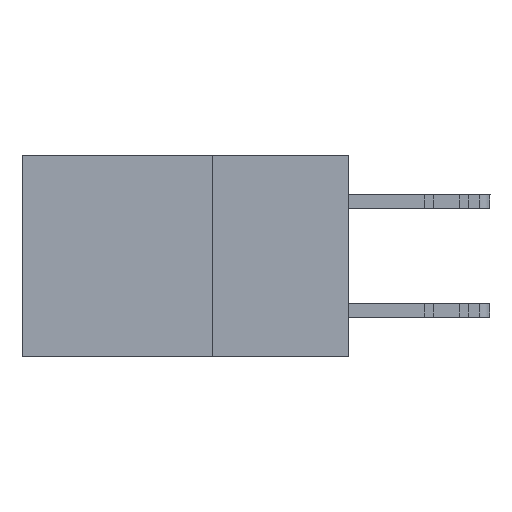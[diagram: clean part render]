
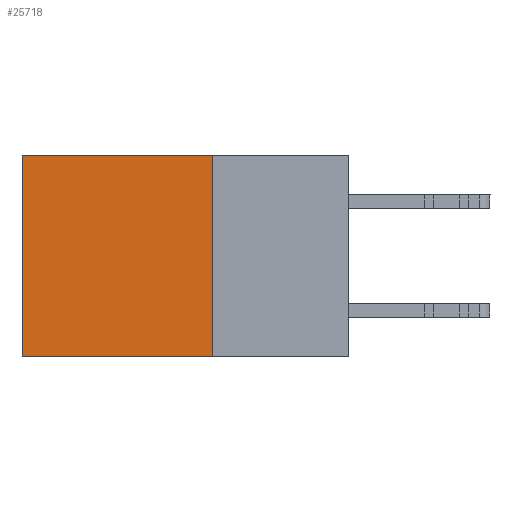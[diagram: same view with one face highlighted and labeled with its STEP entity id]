
A CAD part, left-side view. The second image highlights one B-rep face of the part: STEP entity #25718.
In plain terms, the highlighted planar face has unit normal (-1, 0, 0).
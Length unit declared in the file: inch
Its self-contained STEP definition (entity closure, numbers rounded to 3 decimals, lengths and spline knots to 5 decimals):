
#1016 = DIRECTION ( 'NONE',  ( 0., 0., -1. ) ) ;
#1740 = LINE ( 'NONE', #15560, #11359 ) ;
#2444 = EDGE_CURVE ( 'NONE', #27119, #6983, #7202, .T. ) ;
#3487 = DIRECTION ( 'NONE',  ( 0., 0., -1. ) ) ;
#3711 = ORIENTED_EDGE ( 'NONE', *, *, #20367, .T. ) ;
#4705 = EDGE_CURVE ( 'NONE', #25861, #27119, #5839, .T. ) ;
#5003 = FACE_OUTER_BOUND ( 'NONE', #18993, .T. ) ;
#5608 = VECTOR ( 'NONE', #3487, 39.37008 ) ;
#5630 = CARTESIAN_POINT ( 'NONE',  ( 0.298, 0.6, -0.37 ) ) ;
#5839 = LINE ( 'NONE', #16760, #5608 ) ;
#6544 = CARTESIAN_POINT ( 'NONE',  ( 0.298, 0.6, 0. ) ) ;
#6946 = CARTESIAN_POINT ( 'NONE',  ( 0.298, 0.25, 0. ) ) ;
#6983 = VERTEX_POINT ( 'NONE', #5630 ) ;
#7202 = LINE ( 'NONE', #20782, #8450 ) ;
#7620 = LINE ( 'NONE', #20776, #29014 ) ;
#8450 = VECTOR ( 'NONE', #11633, 39.37008 ) ;
#9418 = ORIENTED_EDGE ( 'NONE', *, *, #4705, .F. ) ;
#9603 = DIRECTION ( 'NONE',  ( 1., 0., 0. ) ) ;
#11330 = VERTEX_POINT ( 'NONE', #6544 ) ;
#11359 = VECTOR ( 'NONE', #13478, 39.37008 ) ;
#11633 = DIRECTION ( 'NONE',  ( 0., 1., 0. ) ) ;
#12542 = CARTESIAN_POINT ( 'NONE',  ( 0.298, 0.25, 0. ) ) ;
#13478 = DIRECTION ( 'NONE',  ( 0., 1., 0. ) ) ;
#14156 = PLANE ( 'NONE',  #19037 ) ;
#15560 = CARTESIAN_POINT ( 'NONE',  ( 0.298, 0.25, 0. ) ) ;
#16760 = CARTESIAN_POINT ( 'NONE',  ( 0.298, 0.25, 0. ) ) ;
#17279 = EDGE_CURVE ( 'NONE', #11330, #6983, #7620, .T. ) ;
#18294 = DIRECTION ( 'NONE',  ( 0., 0., -1. ) ) ;
#18993 = EDGE_LOOP ( 'NONE', ( #23774, #22935, #9418, #3711 ) ) ;
#19037 = AXIS2_PLACEMENT_3D ( 'NONE', #6946, #9603, #18294 ) ;
#20367 = EDGE_CURVE ( 'NONE', #25861, #11330, #1740, .T. ) ;
#20776 = CARTESIAN_POINT ( 'NONE',  ( 0.298, 0.6, 0. ) ) ;
#20782 = CARTESIAN_POINT ( 'NONE',  ( 0.298, 0.25, -0.37 ) ) ;
#22935 = ORIENTED_EDGE ( 'NONE', *, *, #2444, .F. ) ;
#23252 = CARTESIAN_POINT ( 'NONE',  ( 0.298, 0.25, -0.37 ) ) ;
#23774 = ORIENTED_EDGE ( 'NONE', *, *, #17279, .T. ) ;
#25718 = ADVANCED_FACE ( 'NONE', ( #5003 ), #14156, .F. ) ;
#25861 = VERTEX_POINT ( 'NONE', #12542 ) ;
#27119 = VERTEX_POINT ( 'NONE', #23252 ) ;
#29014 = VECTOR ( 'NONE', #1016, 39.37008 ) ;
